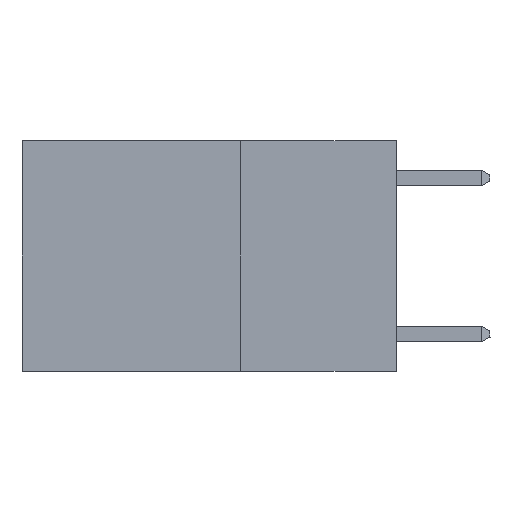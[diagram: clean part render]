
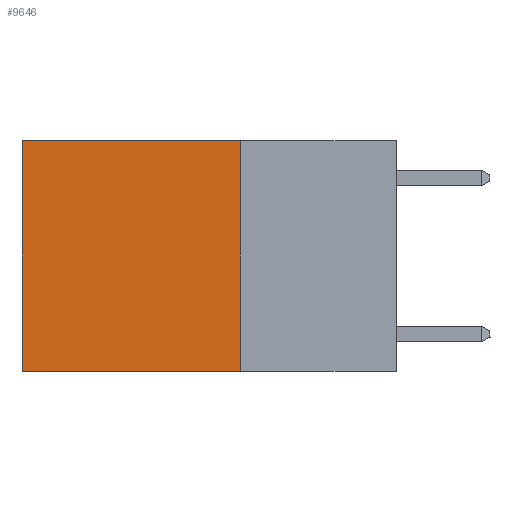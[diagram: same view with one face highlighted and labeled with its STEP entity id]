
A CAD part, left-side view. The second image highlights one B-rep face of the part: STEP entity #9646.
In plain terms, the highlighted planar face has unit normal (-1, 0, 0).
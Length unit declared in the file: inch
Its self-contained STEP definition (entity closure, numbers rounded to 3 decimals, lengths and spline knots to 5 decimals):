
#373 = VERTEX_POINT ( 'NONE', #8153 ) ;
#607 = FACE_OUTER_BOUND ( 'NONE', #2731, .T. ) ;
#781 = ORIENTED_EDGE ( 'NONE', *, *, #8026, .F. ) ;
#992 = VECTOR ( 'NONE', #9128, 39.37008 ) ;
#1310 = LINE ( 'NONE', #10006, #992 ) ;
#2131 = CARTESIAN_POINT ( 'NONE',  ( 0.2625, 0.25, 0. ) ) ;
#2354 = ORIENTED_EDGE ( 'NONE', *, *, #5827, .F. ) ;
#2731 = EDGE_LOOP ( 'NONE', ( #11229, #2354, #781, #9195 ) ) ;
#3027 = VERTEX_POINT ( 'NONE', #7052 ) ;
#3673 = DIRECTION ( 'NONE',  ( 0., 0., -1. ) ) ;
#4487 = CARTESIAN_POINT ( 'NONE',  ( 0.2625, 0.25, 0. ) ) ;
#4925 = AXIS2_PLACEMENT_3D ( 'NONE', #4487, #5456, #11565 ) ;
#5286 = VECTOR ( 'NONE', #8734, 39.37008 ) ;
#5456 = DIRECTION ( 'NONE',  ( 1., 0., 0. ) ) ;
#5495 = PLANE ( 'NONE',  #4925 ) ;
#5501 = EDGE_CURVE ( 'NONE', #7584, #6044, #7667, .T. ) ;
#5827 = EDGE_CURVE ( 'NONE', #373, #6044, #1310, .T. ) ;
#6044 = VERTEX_POINT ( 'NONE', #11156 ) ;
#6199 = LINE ( 'NONE', #2131, #10813 ) ;
#7052 = CARTESIAN_POINT ( 'NONE',  ( 0.2625, 0.25, 0. ) ) ;
#7488 = CARTESIAN_POINT ( 'NONE',  ( 0.2625, 0.6, 0. ) ) ;
#7584 = VERTEX_POINT ( 'NONE', #9032 ) ;
#7667 = LINE ( 'NONE', #7488, #11846 ) ;
#7733 = LINE ( 'NONE', #10392, #5286 ) ;
#8026 = EDGE_CURVE ( 'NONE', #3027, #373, #6199, .T. ) ;
#8153 = CARTESIAN_POINT ( 'NONE',  ( 0.2625, 0.25, -0.37 ) ) ;
#8734 = DIRECTION ( 'NONE',  ( 0., 1., 0. ) ) ;
#8835 = DIRECTION ( 'NONE',  ( 0., 0., -1. ) ) ;
#9032 = CARTESIAN_POINT ( 'NONE',  ( 0.2625, 0.6, 0. ) ) ;
#9128 = DIRECTION ( 'NONE',  ( 0., 1., 0. ) ) ;
#9195 = ORIENTED_EDGE ( 'NONE', *, *, #10218, .T. ) ;
#9646 = ADVANCED_FACE ( 'NONE', ( #607 ), #5495, .F. ) ;
#10006 = CARTESIAN_POINT ( 'NONE',  ( 0.2625, 0.25, -0.37 ) ) ;
#10218 = EDGE_CURVE ( 'NONE', #3027, #7584, #7733, .T. ) ;
#10392 = CARTESIAN_POINT ( 'NONE',  ( 0.2625, 0.25, 0. ) ) ;
#10813 = VECTOR ( 'NONE', #8835, 39.37008 ) ;
#11156 = CARTESIAN_POINT ( 'NONE',  ( 0.2625, 0.6, -0.37 ) ) ;
#11229 = ORIENTED_EDGE ( 'NONE', *, *, #5501, .T. ) ;
#11565 = DIRECTION ( 'NONE',  ( 0., 0., -1. ) ) ;
#11846 = VECTOR ( 'NONE', #3673, 39.37008 ) ;
